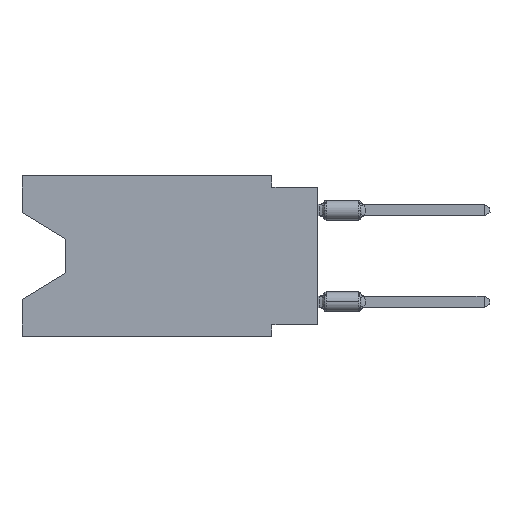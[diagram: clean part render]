
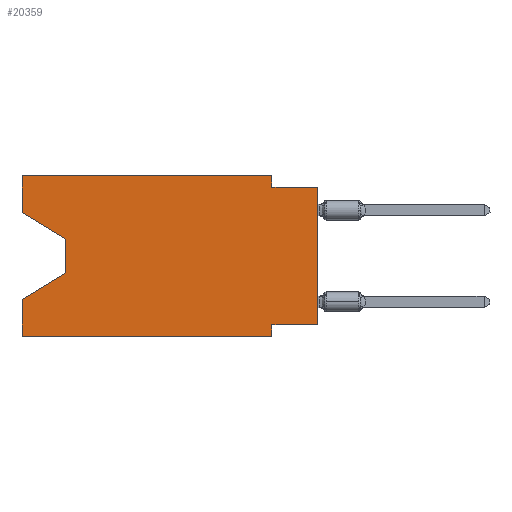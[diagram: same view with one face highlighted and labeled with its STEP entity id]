
A CAD part, left-side view. The second image highlights one B-rep face of the part: STEP entity #20359.
In plain terms, the highlighted planar face has unit normal (-1, 0, 0).
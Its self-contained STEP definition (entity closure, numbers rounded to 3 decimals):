
#184 = VERTEX_POINT ( 'NONE', #15000 ) ;
#480 = DIRECTION ( 'NONE',  ( 0., 0., -1. ) ) ;
#1181 = ORIENTED_EDGE ( 'NONE', *, *, #1924, .F. ) ;
#1184 = EDGE_CURVE ( 'NONE', #3961, #1497, #21100, .T. ) ;
#1497 = VERTEX_POINT ( 'NONE', #16614 ) ;
#1831 = VERTEX_POINT ( 'NONE', #2075 ) ;
#1861 = EDGE_CURVE ( 'NONE', #8668, #2973, #2550, .T. ) ;
#1924 = EDGE_CURVE ( 'NONE', #184, #1831, #4290, .T. ) ;
#2044 = CARTESIAN_POINT ( 'NONE',  ( 0., 2.54, -8.89 ) ) ;
#2075 = CARTESIAN_POINT ( 'NONE',  ( 0., 2.54, -0.635 ) ) ;
#2094 = LINE ( 'NONE', #9210, #7462 ) ;
#2411 = LINE ( 'NONE', #18727, #18742 ) ;
#2550 = LINE ( 'NONE', #8219, #18513 ) ;
#2670 = DIRECTION ( 'NONE',  ( 0., 0., 1. ) ) ;
#2894 = LINE ( 'NONE', #14087, #15626 ) ;
#2973 = VERTEX_POINT ( 'NONE', #10716 ) ;
#3236 = ORIENTED_EDGE ( 'NONE', *, *, #24128, .F. ) ;
#3339 = DIRECTION ( 'NONE',  ( 0., 0., -1. ) ) ;
#3381 = DIRECTION ( 'NONE',  ( 0., 0., 1. ) ) ;
#3604 = VERTEX_POINT ( 'NONE', #20953 ) ;
#3961 = VERTEX_POINT ( 'NONE', #16966 ) ;
#4134 = VECTOR ( 'NONE', #20366, 1000. ) ;
#4215 = EDGE_LOOP ( 'NONE', ( #13689, #11724, #11000, #3236, #4578, #20639, #9823, #22099, #10013, #1181, #20060, #4634 ) ) ;
#4290 = LINE ( 'NONE', #13623, #8713 ) ;
#4384 = DIRECTION ( 'NONE',  ( 0., 0., -1. ) ) ;
#4578 = ORIENTED_EDGE ( 'NONE', *, *, #8470, .T. ) ;
#4634 = ORIENTED_EDGE ( 'NONE', *, *, #16964, .F. ) ;
#4740 = EDGE_CURVE ( 'NONE', #16621, #8668, #16655, .T. ) ;
#6511 = CARTESIAN_POINT ( 'NONE',  ( 0., 16.383, -2.038 ) ) ;
#6729 = LINE ( 'NONE', #8326, #18854 ) ;
#7035 = FACE_OUTER_BOUND ( 'NONE', #4215, .T. ) ;
#7462 = VECTOR ( 'NONE', #16830, 1000. ) ;
#7977 = DIRECTION ( 'NONE',  ( 0., 0.855, -0.519 ) ) ;
#8219 = CARTESIAN_POINT ( 'NONE',  ( 0., 13.97, -5.385 ) ) ;
#8326 = CARTESIAN_POINT ( 'NONE',  ( 0., 16.383, 0. ) ) ;
#8470 = EDGE_CURVE ( 'NONE', #19829, #1497, #2894, .T. ) ;
#8668 = VERTEX_POINT ( 'NONE', #14442 ) ;
#8713 = VECTOR ( 'NONE', #480, 1000. ) ;
#8872 = DIRECTION ( 'NONE',  ( 0., 0., 1. ) ) ;
#9210 = CARTESIAN_POINT ( 'NONE',  ( 0., 16.383, 0. ) ) ;
#9669 = EDGE_CURVE ( 'NONE', #10002, #184, #2094, .T. ) ;
#9823 = ORIENTED_EDGE ( 'NONE', *, *, #13553, .F. ) ;
#10002 = VERTEX_POINT ( 'NONE', #16902 ) ;
#10013 = ORIENTED_EDGE ( 'NONE', *, *, #13849, .F. ) ;
#10224 = VECTOR ( 'NONE', #8872, 1000. ) ;
#10398 = CARTESIAN_POINT ( 'NONE',  ( 0., 0., -8.255 ) ) ;
#10716 = CARTESIAN_POINT ( 'NONE',  ( 0., 16.383, -6.852 ) ) ;
#10964 = VECTOR ( 'NONE', #21517, 1000. ) ;
#11000 = ORIENTED_EDGE ( 'NONE', *, *, #1861, .T. ) ;
#11724 = ORIENTED_EDGE ( 'NONE', *, *, #4740, .T. ) ;
#12066 = CARTESIAN_POINT ( 'NONE',  ( 0., 0., -0.635 ) ) ;
#12492 = DIRECTION ( 'NONE',  ( 0., 1., 0. ) ) ;
#12619 = CARTESIAN_POINT ( 'NONE',  ( 0., 0., 0. ) ) ;
#12692 = DIRECTION ( 'NONE',  ( 1., 0., 0. ) ) ;
#12852 = LINE ( 'NONE', #12619, #22720 ) ;
#13213 = DIRECTION ( 'NONE',  ( 0., -1., 0. ) ) ;
#13553 = EDGE_CURVE ( 'NONE', #3604, #3961, #15595, .T. ) ;
#13623 = CARTESIAN_POINT ( 'NONE',  ( 0., 2.54, 0. ) ) ;
#13689 = ORIENTED_EDGE ( 'NONE', *, *, #15981, .T. ) ;
#13766 = EDGE_CURVE ( 'NONE', #3604, #23299, #12852, .T. ) ;
#13849 = EDGE_CURVE ( 'NONE', #1831, #23299, #2411, .T. ) ;
#14087 = CARTESIAN_POINT ( 'NONE',  ( 0., 16.383, -8.89 ) ) ;
#14442 = CARTESIAN_POINT ( 'NONE',  ( 0., 13.97, -5.385 ) ) ;
#14533 = PLANE ( 'NONE',  #23862 ) ;
#15000 = CARTESIAN_POINT ( 'NONE',  ( 0., 2.54, 0. ) ) ;
#15595 = LINE ( 'NONE', #10398, #19524 ) ;
#15626 = VECTOR ( 'NONE', #15805, 1000. ) ;
#15805 = DIRECTION ( 'NONE',  ( 0., -1., 0. ) ) ;
#15981 = EDGE_CURVE ( 'NONE', #23981, #16621, #23377, .T. ) ;
#16421 = CARTESIAN_POINT ( 'NONE',  ( 0., 13.97, -3.505 ) ) ;
#16614 = CARTESIAN_POINT ( 'NONE',  ( 0., 2.54, -8.89 ) ) ;
#16621 = VERTEX_POINT ( 'NONE', #16889 ) ;
#16655 = LINE ( 'NONE', #16421, #4134 ) ;
#16830 = DIRECTION ( 'NONE',  ( 0., -1., 0. ) ) ;
#16889 = CARTESIAN_POINT ( 'NONE',  ( 0., 13.97, -3.505 ) ) ;
#16902 = CARTESIAN_POINT ( 'NONE',  ( 0., 16.383, 0. ) ) ;
#16964 = EDGE_CURVE ( 'NONE', #23981, #10002, #18454, .T. ) ;
#16966 = CARTESIAN_POINT ( 'NONE',  ( 0., 2.54, -8.255 ) ) ;
#17175 = CARTESIAN_POINT ( 'NONE',  ( 0., 16.383, -2.038 ) ) ;
#18202 = CARTESIAN_POINT ( 'NONE',  ( 0., 16.383, 0. ) ) ;
#18454 = LINE ( 'NONE', #18202, #10224 ) ;
#18513 = VECTOR ( 'NONE', #7977, 1000. ) ;
#18727 = CARTESIAN_POINT ( 'NONE',  ( 0., 0., -0.635 ) ) ;
#18742 = VECTOR ( 'NONE', #13213, 1000. ) ;
#18854 = VECTOR ( 'NONE', #2670, 1000. ) ;
#19121 = VECTOR ( 'NONE', #4384, 1000. ) ;
#19524 = VECTOR ( 'NONE', #12492, 1000. ) ;
#19829 = VERTEX_POINT ( 'NONE', #23248 ) ;
#20060 = ORIENTED_EDGE ( 'NONE', *, *, #9669, .F. ) ;
#20359 = ADVANCED_FACE ( 'NONE', ( #7035 ), #14533, .F. ) ;
#20366 = DIRECTION ( 'NONE',  ( 0., 0., -1. ) ) ;
#20639 = ORIENTED_EDGE ( 'NONE', *, *, #1184, .F. ) ;
#20953 = CARTESIAN_POINT ( 'NONE',  ( 0., 0., -8.255 ) ) ;
#21100 = LINE ( 'NONE', #2044, #19121 ) ;
#21517 = DIRECTION ( 'NONE',  ( 0., -0.855, -0.519 ) ) ;
#22050 = CARTESIAN_POINT ( 'NONE',  ( 0., 16.383, 0. ) ) ;
#22099 = ORIENTED_EDGE ( 'NONE', *, *, #13766, .T. ) ;
#22720 = VECTOR ( 'NONE', #3381, 1000. ) ;
#23248 = CARTESIAN_POINT ( 'NONE',  ( 0., 16.383, -8.89 ) ) ;
#23299 = VERTEX_POINT ( 'NONE', #12066 ) ;
#23377 = LINE ( 'NONE', #6511, #10964 ) ;
#23862 = AXIS2_PLACEMENT_3D ( 'NONE', #22050, #12692, #3339 ) ;
#23981 = VERTEX_POINT ( 'NONE', #17175 ) ;
#24128 = EDGE_CURVE ( 'NONE', #19829, #2973, #6729, .T. ) ;
